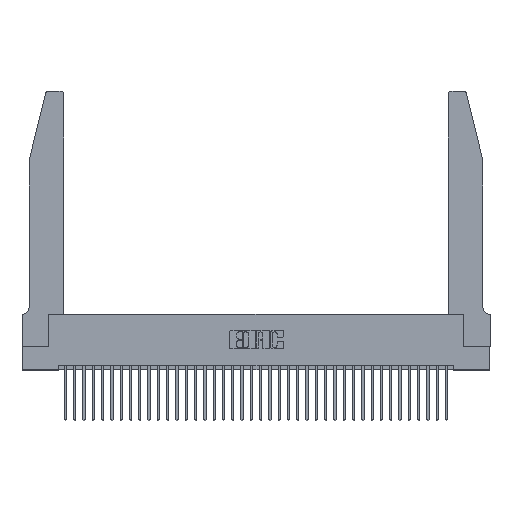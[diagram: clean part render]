
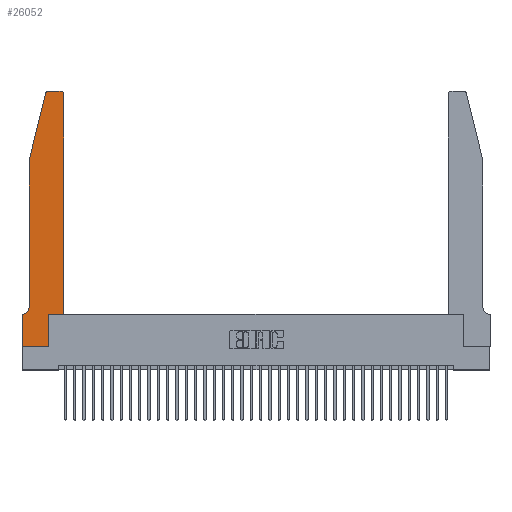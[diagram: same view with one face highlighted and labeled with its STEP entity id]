
A CAD part, top view. The second image highlights one B-rep face of the part: STEP entity #26052.
In plain terms, the highlighted planar face has unit normal (0, 0, 1).
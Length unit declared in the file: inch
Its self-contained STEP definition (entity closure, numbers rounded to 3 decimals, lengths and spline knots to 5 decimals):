
#730 = VERTEX_POINT ( 'NONE', #2477 ) ;
#785 = DIRECTION ( 'NONE',  ( -1., 0., 0. ) ) ;
#799 = ORIENTED_EDGE ( 'NONE', *, *, #34255, .T. ) ;
#1369 = CARTESIAN_POINT ( 'NONE',  ( 0.2865, 0., 0.37 ) ) ;
#1761 = ORIENTED_EDGE ( 'NONE', *, *, #16829, .T. ) ;
#1882 = CARTESIAN_POINT ( 'NONE',  ( 0.0755, 2., 0.37 ) ) ;
#1964 = LINE ( 'NONE', #14365, #6504 ) ;
#2045 = CARTESIAN_POINT ( 'NONE',  ( 0.4505, 0.35, 0.37 ) ) ;
#2445 = DIRECTION ( 'NONE',  ( 0., -1., 0. ) ) ;
#2477 = CARTESIAN_POINT ( 'NONE',  ( 0.4205, 2.75, 0.37 ) ) ;
#2733 = ORIENTED_EDGE ( 'NONE', *, *, #33627, .T. ) ;
#3462 = EDGE_CURVE ( 'NONE', #27588, #33936, #26899, .T. ) ;
#3812 = ORIENTED_EDGE ( 'NONE', *, *, #20632, .T. ) ;
#4367 = CARTESIAN_POINT ( 'NONE',  ( 0.0055, 0.35, 0.37 ) ) ;
#4730 = DIRECTION ( 'NONE',  ( 0., 1., 0. ) ) ;
#4886 = CIRCLE ( 'NONE', #34210, 0.07 ) ;
#5119 = EDGE_CURVE ( 'NONE', #730, #29328, #10544, .T. ) ;
#6248 = CARTESIAN_POINT ( 'NONE',  ( 0., 0.35, 0.37 ) ) ;
#6504 = VECTOR ( 'NONE', #20350, 39.37008 ) ;
#6645 = CIRCLE ( 'NONE', #34567, 0.03 ) ;
#6739 = CARTESIAN_POINT ( 'NONE',  ( 0.25487, 2.72718, 0.37 ) ) ;
#6915 = VERTEX_POINT ( 'NONE', #4367 ) ;
#7070 = CARTESIAN_POINT ( 'NONE',  ( 0.4505, 2.72, 0.37 ) ) ;
#7185 = CARTESIAN_POINT ( 'NONE',  ( 0.0755, 2., 0.37 ) ) ;
#7373 = EDGE_CURVE ( 'NONE', #32944, #6915, #4886, .T. ) ;
#7896 = EDGE_CURVE ( 'NONE', #6915, #18557, #33094, .T. ) ;
#7974 = DIRECTION ( 'NONE',  ( 0., 0., 1. ) ) ;
#8497 = DIRECTION ( 'NONE',  ( 1., 0., 0. ) ) ;
#8671 = ORIENTED_EDGE ( 'NONE', *, *, #3462, .T. ) ;
#8923 = CARTESIAN_POINT ( 'NONE',  ( 0., 0.35, 0.37 ) ) ;
#9464 = CARTESIAN_POINT ( 'NONE',  ( 0.2605, 2.75, 0.37 ) ) ;
#10544 = LINE ( 'NONE', #9464, #20559 ) ;
#10722 = DIRECTION ( 'NONE',  ( 1., 0., 0. ) ) ;
#11796 = EDGE_LOOP ( 'NONE', ( #12448, #26746, #3812, #1761, #33416, #12223, #23652, #20190, #30275, #2733, #8671, #799 ) ) ;
#12223 = ORIENTED_EDGE ( 'NONE', *, *, #7896, .T. ) ;
#12448 = ORIENTED_EDGE ( 'NONE', *, *, #5119, .T. ) ;
#13309 = LINE ( 'NONE', #19989, #34687 ) ;
#13768 = CARTESIAN_POINT ( 'NONE',  ( 0.4505, 0.35, 0.37 ) ) ;
#13930 = VECTOR ( 'NONE', #27814, 39.37008 ) ;
#14247 = CARTESIAN_POINT ( 'NONE',  ( 0., 0., 0.37 ) ) ;
#14365 = CARTESIAN_POINT ( 'NONE',  ( 0.2865, 0.35, 0.37 ) ) ;
#14734 = AXIS2_PLACEMENT_3D ( 'NONE', #8923, #20649, #23579 ) ;
#15003 = FACE_OUTER_BOUND ( 'NONE', #11796, .T. ) ;
#15217 = VERTEX_POINT ( 'NONE', #1882 ) ;
#15269 = EDGE_CURVE ( 'NONE', #29328, #30090, #34520, .T. ) ;
#16780 = DIRECTION ( 'NONE',  ( 1., 0., 0. ) ) ;
#16782 = VERTEX_POINT ( 'NONE', #20024 ) ;
#16829 = EDGE_CURVE ( 'NONE', #15217, #32944, #34030, .T. ) ;
#18557 = VERTEX_POINT ( 'NONE', #6248 ) ;
#19085 = CARTESIAN_POINT ( 'NONE',  ( 0.0055, 0.42, 0.37 ) ) ;
#19215 = VECTOR ( 'NONE', #4730, 39.37008 ) ;
#19810 = CARTESIAN_POINT ( 'NONE',  ( 0.0755, 0.42, 0.37 ) ) ;
#19989 = CARTESIAN_POINT ( 'NONE',  ( 0.0755, 2., 0.37 ) ) ;
#20024 = CARTESIAN_POINT ( 'NONE',  ( 0.2865, 0.35, 0.37 ) ) ;
#20190 = ORIENTED_EDGE ( 'NONE', *, *, #26946, .T. ) ;
#20275 = CARTESIAN_POINT ( 'NONE',  ( 0., 0., 0.37 ) ) ;
#20350 = DIRECTION ( 'NONE',  ( 0., 1., 0. ) ) ;
#20559 = VECTOR ( 'NONE', #785, 39.37008 ) ;
#20632 = EDGE_CURVE ( 'NONE', #30090, #15217, #13309, .T. ) ;
#20649 = DIRECTION ( 'NONE',  ( 0., 0., 1. ) ) ;
#21047 = CARTESIAN_POINT ( 'NONE',  ( 0.284, 2.75, 0.37 ) ) ;
#21860 = DIRECTION ( 'NONE',  ( -1., 0., 0. ) ) ;
#22358 = DIRECTION ( 'NONE',  ( -1., 0., 0. ) ) ;
#23122 = CARTESIAN_POINT ( 'NONE',  ( 0.4205, 2.72, 0.37 ) ) ;
#23579 = DIRECTION ( 'NONE',  ( 1., 0., 0. ) ) ;
#23652 = ORIENTED_EDGE ( 'NONE', *, *, #29814, .T. ) ;
#25155 = DIRECTION ( 'NONE',  ( 0., 0., -1. ) ) ;
#25368 = VECTOR ( 'NONE', #21860, 39.37008 ) ;
#26052 = ADVANCED_FACE ( 'NONE', ( #15003 ), #31847, .T. ) ;
#26746 = ORIENTED_EDGE ( 'NONE', *, *, #15269, .T. ) ;
#26899 = LINE ( 'NONE', #2045, #19215 ) ;
#26946 = EDGE_CURVE ( 'NONE', #33028, #28450, #34084, .T. ) ;
#26983 = LINE ( 'NONE', #20275, #35632 ) ;
#27586 = DIRECTION ( 'NONE',  ( 1., 0., 0. ) ) ;
#27588 = VERTEX_POINT ( 'NONE', #34446 ) ;
#27814 = DIRECTION ( 'NONE',  ( 0., -1., 0. ) ) ;
#28114 = CARTESIAN_POINT ( 'NONE',  ( 0.284, 2.72, 0.37 ) ) ;
#28191 = CARTESIAN_POINT ( 'NONE',  ( 0., 0., 0.37 ) ) ;
#28450 = VERTEX_POINT ( 'NONE', #1369 ) ;
#28618 = DIRECTION ( 'NONE',  ( -0.239, -0.971, 0. ) ) ;
#29328 = VERTEX_POINT ( 'NONE', #21047 ) ;
#29814 = EDGE_CURVE ( 'NONE', #18557, #33028, #26983, .T. ) ;
#30090 = VERTEX_POINT ( 'NONE', #6739 ) ;
#30275 = ORIENTED_EDGE ( 'NONE', *, *, #37171, .T. ) ;
#30633 = DIRECTION ( 'NONE',  ( 0., 0., 1. ) ) ;
#31847 = PLANE ( 'NONE',  #14734 ) ;
#32944 = VERTEX_POINT ( 'NONE', #19810 ) ;
#33028 = VERTEX_POINT ( 'NONE', #28191 ) ;
#33094 = LINE ( 'NONE', #33835, #25368 ) ;
#33135 = VECTOR ( 'NONE', #10722, 39.37008 ) ;
#33280 = AXIS2_PLACEMENT_3D ( 'NONE', #28114, #30633, #27586 ) ;
#33416 = ORIENTED_EDGE ( 'NONE', *, *, #7373, .T. ) ;
#33627 = EDGE_CURVE ( 'NONE', #16782, #27588, #34067, .T. ) ;
#33835 = CARTESIAN_POINT ( 'NONE',  ( 0.0755, 0.35, 0.37 ) ) ;
#33936 = VERTEX_POINT ( 'NONE', #7070 ) ;
#34030 = LINE ( 'NONE', #7185, #13930 ) ;
#34067 = LINE ( 'NONE', #13768, #33135 ) ;
#34084 = LINE ( 'NONE', #14247, #36817 ) ;
#34210 = AXIS2_PLACEMENT_3D ( 'NONE', #19085, #25155, #22358 ) ;
#34255 = EDGE_CURVE ( 'NONE', #33936, #730, #6645, .T. ) ;
#34446 = CARTESIAN_POINT ( 'NONE',  ( 0.4505, 0.35, 0.37 ) ) ;
#34520 = CIRCLE ( 'NONE', #33280, 0.03 ) ;
#34567 = AXIS2_PLACEMENT_3D ( 'NONE', #23122, #7974, #16780 ) ;
#34687 = VECTOR ( 'NONE', #28618, 39.37008 ) ;
#35632 = VECTOR ( 'NONE', #2445, 39.37008 ) ;
#36817 = VECTOR ( 'NONE', #8497, 39.37008 ) ;
#37171 = EDGE_CURVE ( 'NONE', #28450, #16782, #1964, .T. ) ;
